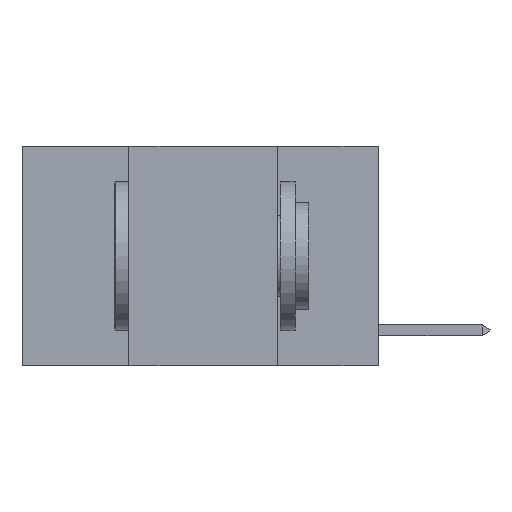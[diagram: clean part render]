
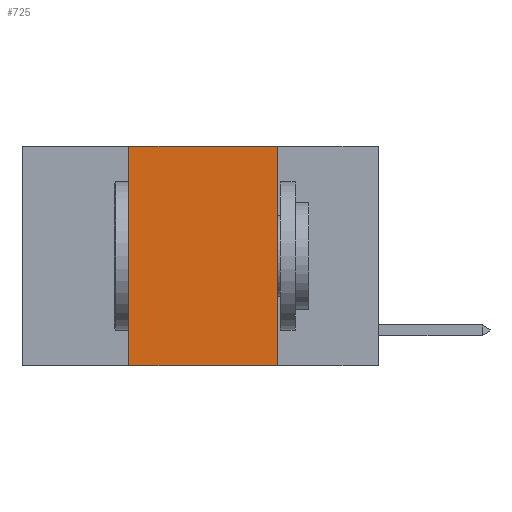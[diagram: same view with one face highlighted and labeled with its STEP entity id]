
A CAD part, left-side view. The second image highlights one B-rep face of the part: STEP entity #725.
In plain terms, the highlighted planar face has unit normal (-1, 0, 0).
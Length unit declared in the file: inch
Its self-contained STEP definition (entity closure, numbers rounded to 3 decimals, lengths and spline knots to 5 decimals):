
#219 = CARTESIAN_POINT ( 'NONE',  ( 0., 0.42, 0. ) ) ;
#725 = ADVANCED_FACE ( 'NONE', ( #4411 ), #12324, .F. ) ;
#1464 = VERTEX_POINT ( 'NONE', #5777 ) ;
#2490 = DIRECTION ( 'NONE',  ( 1., 0., 0. ) ) ;
#4064 = AXIS2_PLACEMENT_3D ( 'NONE', #20175, #2490, #20804 ) ;
#4411 = FACE_OUTER_BOUND ( 'NONE', #8913, .T. ) ;
#4908 = LINE ( 'NONE', #16802, #20838 ) ;
#5777 = CARTESIAN_POINT ( 'NONE',  ( 0., 0.17, -0.37 ) ) ;
#6856 = DIRECTION ( 'NONE',  ( 0., -1., 0. ) ) ;
#7151 = EDGE_CURVE ( 'NONE', #21330, #1464, #13318, .T. ) ;
#8392 = EDGE_CURVE ( 'NONE', #21196, #1464, #4908, .T. ) ;
#8913 = EDGE_LOOP ( 'NONE', ( #15627, #22197, #19612, #23811 ) ) ;
#10376 = EDGE_CURVE ( 'NONE', #21196, #10716, #13655, .T. ) ;
#10716 = VERTEX_POINT ( 'NONE', #11558 ) ;
#11558 = CARTESIAN_POINT ( 'NONE',  ( 0., 0.42, 0. ) ) ;
#11973 = DIRECTION ( 'NONE',  ( 0., 0., 1. ) ) ;
#12250 = LINE ( 'NONE', #20086, #22593 ) ;
#12324 = PLANE ( 'NONE',  #4064 ) ;
#13318 = LINE ( 'NONE', #15881, #24887 ) ;
#13655 = LINE ( 'NONE', #219, #19435 ) ;
#14299 = DIRECTION ( 'NONE',  ( 0., -1., 0. ) ) ;
#15627 = ORIENTED_EDGE ( 'NONE', *, *, #7151, .F. ) ;
#15881 = CARTESIAN_POINT ( 'NONE',  ( 0., 0.17, 0. ) ) ;
#16802 = CARTESIAN_POINT ( 'NONE',  ( 0., 0.6, -0.37 ) ) ;
#18536 = EDGE_CURVE ( 'NONE', #10716, #21330, #12250, .T. ) ;
#18937 = CARTESIAN_POINT ( 'NONE',  ( 0., 0.42, -0.37 ) ) ;
#19435 = VECTOR ( 'NONE', #11973, 39.37008 ) ;
#19612 = ORIENTED_EDGE ( 'NONE', *, *, #10376, .F. ) ;
#19844 = DIRECTION ( 'NONE',  ( 0., 0., -1. ) ) ;
#20086 = CARTESIAN_POINT ( 'NONE',  ( 0., 0.6, 0. ) ) ;
#20175 = CARTESIAN_POINT ( 'NONE',  ( 0., 0.6, 0. ) ) ;
#20490 = CARTESIAN_POINT ( 'NONE',  ( 0., 0.17, 0. ) ) ;
#20804 = DIRECTION ( 'NONE',  ( 0., 0., -1. ) ) ;
#20838 = VECTOR ( 'NONE', #6856, 39.37008 ) ;
#21196 = VERTEX_POINT ( 'NONE', #18937 ) ;
#21330 = VERTEX_POINT ( 'NONE', #20490 ) ;
#22197 = ORIENTED_EDGE ( 'NONE', *, *, #18536, .F. ) ;
#22593 = VECTOR ( 'NONE', #14299, 39.37008 ) ;
#23811 = ORIENTED_EDGE ( 'NONE', *, *, #8392, .T. ) ;
#24887 = VECTOR ( 'NONE', #19844, 39.37008 ) ;
